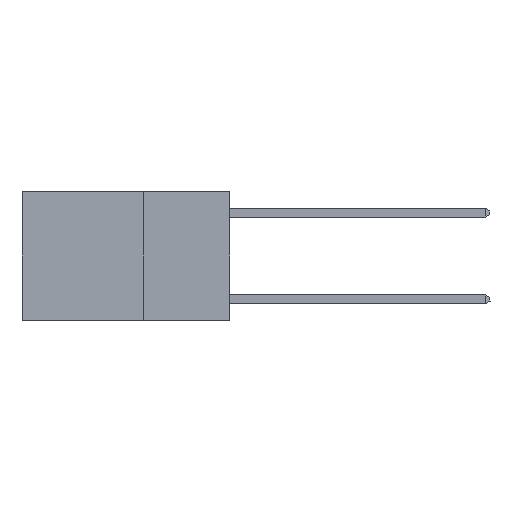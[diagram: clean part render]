
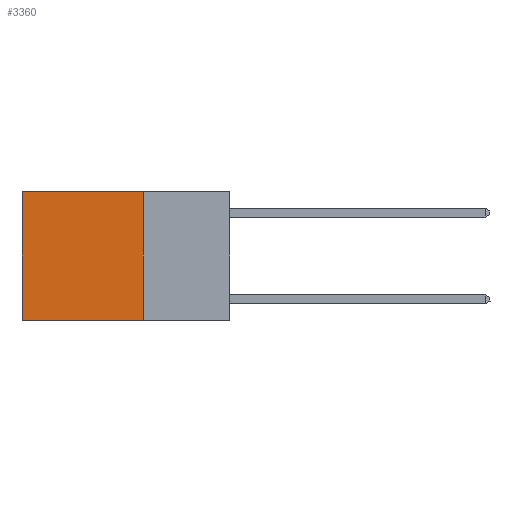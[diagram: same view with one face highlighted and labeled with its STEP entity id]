
A CAD part, left-side view. The second image highlights one B-rep face of the part: STEP entity #3360.
In plain terms, the highlighted planar face has unit normal (-1, 0, 0).
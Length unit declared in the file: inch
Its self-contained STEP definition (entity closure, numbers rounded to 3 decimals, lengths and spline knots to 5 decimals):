
#39 = CARTESIAN_POINT ( 'NONE',  ( 0.2625, 0.25, 0. ) ) ;
#268 = CARTESIAN_POINT ( 'NONE',  ( 0.2625, 0.25, 0. ) ) ;
#324 = ORIENTED_EDGE ( 'NONE', *, *, #5324, .T. ) ;
#328 = LINE ( 'NONE', #12695, #9192 ) ;
#1048 = VERTEX_POINT ( 'NONE', #2417 ) ;
#1327 = PLANE ( 'NONE',  #3526 ) ;
#1910 = VECTOR ( 'NONE', #11847, 39.37008 ) ;
#2417 = CARTESIAN_POINT ( 'NONE',  ( 0.2625, 0.6, 0. ) ) ;
#2483 = ORIENTED_EDGE ( 'NONE', *, *, #6363, .T. ) ;
#3337 = VECTOR ( 'NONE', #4334, 39.37008 ) ;
#3360 = ADVANCED_FACE ( 'NONE', ( #6230 ), #1327, .F. ) ;
#3526 = AXIS2_PLACEMENT_3D ( 'NONE', #268, #4423, #5424 ) ;
#3654 = CARTESIAN_POINT ( 'NONE',  ( 0.2625, 0.6, 0. ) ) ;
#3923 = VERTEX_POINT ( 'NONE', #6331 ) ;
#4067 = ORIENTED_EDGE ( 'NONE', *, *, #10316, .F. ) ;
#4334 = DIRECTION ( 'NONE',  ( 0., 0., -1. ) ) ;
#4423 = DIRECTION ( 'NONE',  ( 1., 0., 0. ) ) ;
#5324 = EDGE_CURVE ( 'NONE', #1048, #9602, #9844, .T. ) ;
#5424 = DIRECTION ( 'NONE',  ( 0., 0., -1. ) ) ;
#5756 = CARTESIAN_POINT ( 'NONE',  ( 0.2625, 0.25, 0. ) ) ;
#6230 = FACE_OUTER_BOUND ( 'NONE', #8728, .T. ) ;
#6331 = CARTESIAN_POINT ( 'NONE',  ( 0.2625, 0.25, -0.37 ) ) ;
#6363 = EDGE_CURVE ( 'NONE', #12967, #1048, #328, .T. ) ;
#8117 = DIRECTION ( 'NONE',  ( 0., 1., 0. ) ) ;
#8728 = EDGE_LOOP ( 'NONE', ( #324, #9550, #4067, #2483 ) ) ;
#9192 = VECTOR ( 'NONE', #11592, 39.37008 ) ;
#9409 = CARTESIAN_POINT ( 'NONE',  ( 0.2625, 0.6, -0.37 ) ) ;
#9515 = LINE ( 'NONE', #39, #3337 ) ;
#9550 = ORIENTED_EDGE ( 'NONE', *, *, #12446, .F. ) ;
#9602 = VERTEX_POINT ( 'NONE', #9409 ) ;
#9844 = LINE ( 'NONE', #3654, #1910 ) ;
#10316 = EDGE_CURVE ( 'NONE', #12967, #3923, #9515, .T. ) ;
#10576 = VECTOR ( 'NONE', #8117, 39.37008 ) ;
#11052 = CARTESIAN_POINT ( 'NONE',  ( 0.2625, 0.25, -0.37 ) ) ;
#11366 = LINE ( 'NONE', #11052, #10576 ) ;
#11592 = DIRECTION ( 'NONE',  ( 0., 1., 0. ) ) ;
#11847 = DIRECTION ( 'NONE',  ( 0., 0., -1. ) ) ;
#12446 = EDGE_CURVE ( 'NONE', #3923, #9602, #11366, .T. ) ;
#12695 = CARTESIAN_POINT ( 'NONE',  ( 0.2625, 0.25, 0. ) ) ;
#12967 = VERTEX_POINT ( 'NONE', #5756 ) ;
